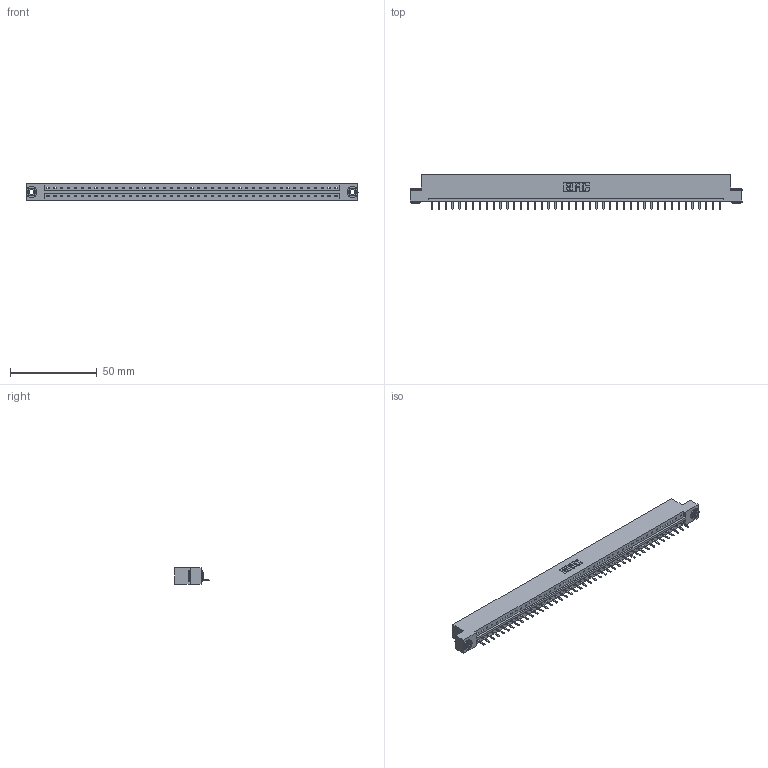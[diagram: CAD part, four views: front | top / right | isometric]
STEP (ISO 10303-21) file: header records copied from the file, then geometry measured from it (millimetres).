
FILE_DESCRIPTION (( 'STEP AP203' ), '1' );
FILE_NAME ('333-043-520-103.STEP', '2018-08-03T19:59:44', ( '' ), ( '' ), 'SwSTEP 2.0', 'SolidWorks 2016', '' );
FILE_SCHEMA (( 'CONFIG_CONTROL_DESIGN' ));
Length unit declared in the file: inch
Products named in the file (4): 333 Part_Flush - .156 Dia - TH; 345-292-001_345-293-120; 345-250-002_345-250-002-102; 333-043-520-103
Assembly tree (46 placements, depth 2):
  333-043-520-103
    333 Part_Flush - .156 Dia - TH
    345-292-001_345-293-120  x43
    345-250-002_345-250-002-102  x2
Bounding box: 191.92 x 20.02 x 9.4 mm (x, y, z)
Volume: 19217.1 mm3; surface area: 20592.9 mm2
Topology: 46 solids, 46 shells, 2818 faces, 8299 edges, 5414 vertices
Faces by surface type: plane 1972, cylinder 838, cone 8
Entity records: 26922 total; most frequent: CARTESIAN_POINT 4634, ORIENTED_EDGE 4594, DIRECTION 3929, EDGE_CURVE 2297, LINE 2141, VECTOR 2141, VERTEX_POINT 1526, AXIS2_PLACEMENT_3D 894
